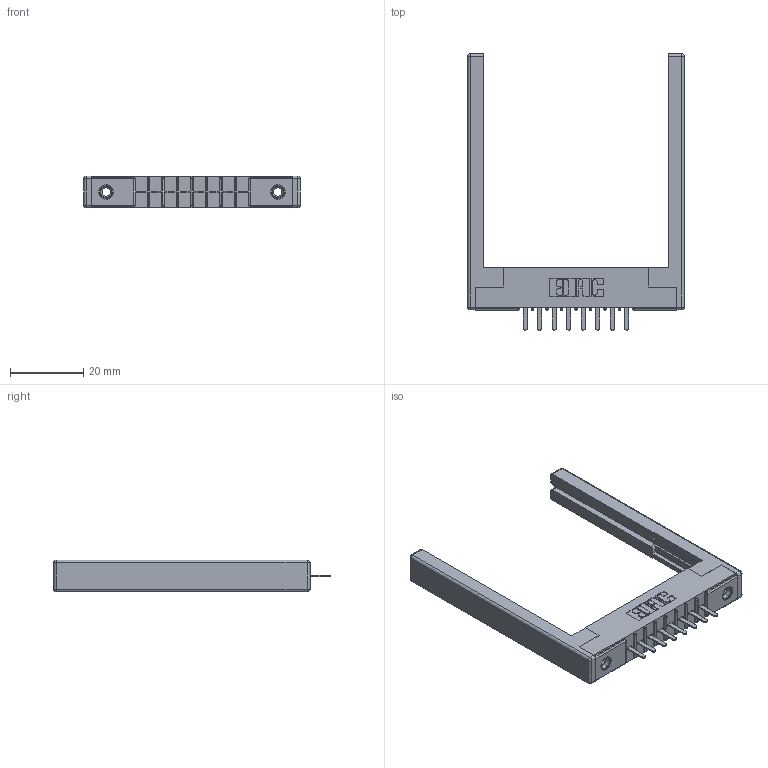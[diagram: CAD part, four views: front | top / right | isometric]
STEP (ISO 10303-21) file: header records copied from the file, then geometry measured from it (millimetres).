
FILE_DESCRIPTION (( 'STEP AP203' ), '1' );
FILE_NAME ('356-008-520-168.STEP', '2018-07-31T06:38:25', ( '' ), ( '' ), 'SwSTEP 2.0', 'SolidWorks 2016', '' );
FILE_SCHEMA (( 'CONFIG_CONTROL_DESIGN' ));
Length unit declared in the file: inch
Products named in the file (5): 356-008-520-168; 306 Part_.156 Dia; 306-290-001_120; 345-250-001_345-250-001-102; 307-220-068
Assembly tree (13 placements, depth 2):
  356-008-520-168
    306 Part_.156 Dia
    306-290-001_120  x8
    345-250-001_345-250-001-102  x2
    307-220-068  x2
Bounding box: 59.13 x 75.41 x 8.71 mm (x, y, z)
Volume: 8527.8 mm3; surface area: 9565.4 mm2
Topology: 13 solids, 13 shells, 830 faces, 2282 edges, 1456 vertices
Faces by surface type: plane 532, cylinder 242, sphere 40, cone 12, torus 4
Entity records: 14580 total; most frequent: CARTESIAN_POINT 2408, DIRECTION 2391, ORIENTED_EDGE 2374, EDGE_CURVE 1187, VECTOR 905, LINE 905, VERTEX_POINT 760, AXIS2_PLACEMENT_3D 743
